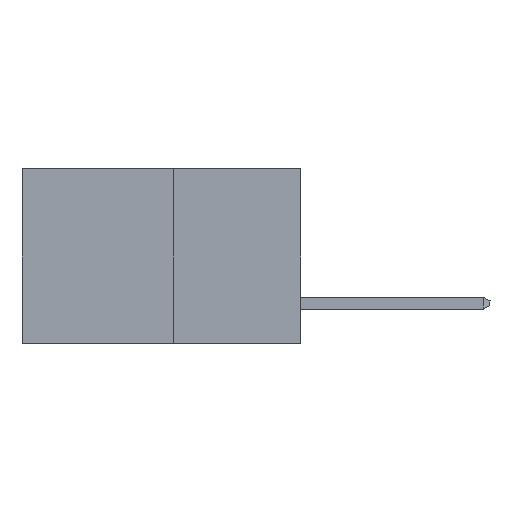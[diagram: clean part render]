
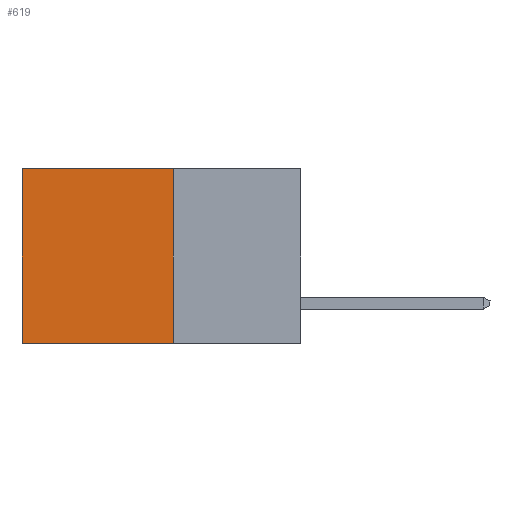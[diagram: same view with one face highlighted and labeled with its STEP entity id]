
A CAD part, left-side view. The second image highlights one B-rep face of the part: STEP entity #619.
In plain terms, the highlighted planar face has unit normal (-1, 0, 0).
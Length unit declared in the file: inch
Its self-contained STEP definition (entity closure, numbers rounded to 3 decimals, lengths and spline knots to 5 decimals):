
#619 = ADVANCED_FACE ( 'NONE', ( #15051 ), #15133, .F. ) ;
#1666 = ORIENTED_EDGE ( 'NONE', *, *, #2923, .T. ) ;
#2257 = VECTOR ( 'NONE', #6107, 39.37008 ) ;
#2390 = VERTEX_POINT ( 'NONE', #4554 ) ;
#2619 = ORIENTED_EDGE ( 'NONE', *, *, #18608, .F. ) ;
#2923 = EDGE_CURVE ( 'NONE', #6859, #2390, #5841, .T. ) ;
#3258 = CARTESIAN_POINT ( 'NONE',  ( 0.277, 0.27, -0.37 ) ) ;
#4414 = EDGE_CURVE ( 'NONE', #8619, #10565, #13383, .T. ) ;
#4554 = CARTESIAN_POINT ( 'NONE',  ( 0.277, 0.59, 0. ) ) ;
#5002 = VECTOR ( 'NONE', #16720, 39.37008 ) ;
#5048 = EDGE_CURVE ( 'NONE', #2390, #10565, #13572, .T. ) ;
#5634 = DIRECTION ( 'NONE',  ( 0., 0., -1. ) ) ;
#5841 = LINE ( 'NONE', #12954, #2257 ) ;
#5885 = CARTESIAN_POINT ( 'NONE',  ( 0.277, 0.59, -0.37 ) ) ;
#6107 = DIRECTION ( 'NONE',  ( 0., 1., 0. ) ) ;
#6859 = VERTEX_POINT ( 'NONE', #14098 ) ;
#7252 = ORIENTED_EDGE ( 'NONE', *, *, #5048, .T. ) ;
#8087 = CARTESIAN_POINT ( 'NONE',  ( 0.277, 0.59, -0.37 ) ) ;
#8213 = AXIS2_PLACEMENT_3D ( 'NONE', #15197, #16370, #16356 ) ;
#8314 = DIRECTION ( 'NONE',  ( 0., 1., 0. ) ) ;
#8619 = VERTEX_POINT ( 'NONE', #3258 ) ;
#9001 = LINE ( 'NONE', #12234, #5002 ) ;
#10565 = VERTEX_POINT ( 'NONE', #8087 ) ;
#12234 = CARTESIAN_POINT ( 'NONE',  ( 0.277, 0.27, -0.37 ) ) ;
#12954 = CARTESIAN_POINT ( 'NONE',  ( 0.277, 0.27, 0. ) ) ;
#13121 = VECTOR ( 'NONE', #5634, 39.37008 ) ;
#13383 = LINE ( 'NONE', #19102, #17717 ) ;
#13572 = LINE ( 'NONE', #5885, #13121 ) ;
#14098 = CARTESIAN_POINT ( 'NONE',  ( 0.277, 0.27, 0. ) ) ;
#14537 = EDGE_LOOP ( 'NONE', ( #7252, #15778, #2619, #1666 ) ) ;
#15051 = FACE_OUTER_BOUND ( 'NONE', #14537, .T. ) ;
#15133 = PLANE ( 'NONE',  #8213 ) ;
#15197 = CARTESIAN_POINT ( 'NONE',  ( 0.277, 0.27, -0.37 ) ) ;
#15778 = ORIENTED_EDGE ( 'NONE', *, *, #4414, .F. ) ;
#16356 = DIRECTION ( 'NONE',  ( 0., 0., -1. ) ) ;
#16370 = DIRECTION ( 'NONE',  ( 1., 0., 0. ) ) ;
#16720 = DIRECTION ( 'NONE',  ( 0., 0., -1. ) ) ;
#17717 = VECTOR ( 'NONE', #8314, 39.37008 ) ;
#18608 = EDGE_CURVE ( 'NONE', #6859, #8619, #9001, .T. ) ;
#19102 = CARTESIAN_POINT ( 'NONE',  ( 0.277, 0.27, -0.37 ) ) ;
